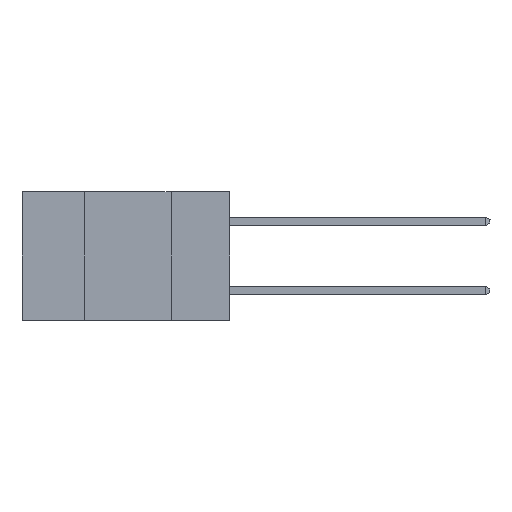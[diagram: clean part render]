
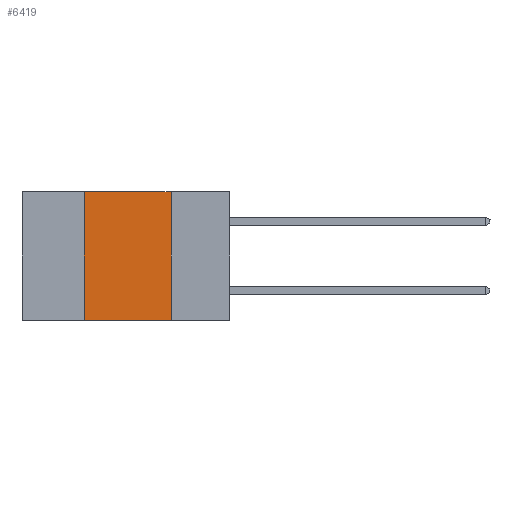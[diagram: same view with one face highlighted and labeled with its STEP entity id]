
A CAD part, left-side view. The second image highlights one B-rep face of the part: STEP entity #6419.
In plain terms, the highlighted planar face has unit normal (-1, 0, 0).
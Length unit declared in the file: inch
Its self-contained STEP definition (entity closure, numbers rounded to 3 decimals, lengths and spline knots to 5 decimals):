
#238 = EDGE_LOOP ( 'NONE', ( #22168, #12930, #23128, #16556 ) ) ;
#379 = LINE ( 'NONE', #8680, #2944 ) ;
#1309 = CARTESIAN_POINT ( 'NONE',  ( 0., 0.42, -0.37 ) ) ;
#1664 = CARTESIAN_POINT ( 'NONE',  ( 0., 0.17, -0.37 ) ) ;
#2242 = EDGE_CURVE ( 'NONE', #11374, #11615, #15884, .T. ) ;
#2944 = VECTOR ( 'NONE', #8531, 39.37008 ) ;
#3778 = DIRECTION ( 'NONE',  ( 0., -1., 0. ) ) ;
#4526 = EDGE_CURVE ( 'NONE', #20622, #18560, #5500, .T. ) ;
#4681 = DIRECTION ( 'NONE',  ( 0., 0., 1. ) ) ;
#5164 = DIRECTION ( 'NONE',  ( 0., 0., -1. ) ) ;
#5500 = LINE ( 'NONE', #20029, #12405 ) ;
#6259 = CARTESIAN_POINT ( 'NONE',  ( 0., 0.17, 0. ) ) ;
#6419 = ADVANCED_FACE ( 'NONE', ( #12013 ), #8944, .F. ) ;
#6427 = LINE ( 'NONE', #17594, #14457 ) ;
#8531 = DIRECTION ( 'NONE',  ( 0., 0., -1. ) ) ;
#8680 = CARTESIAN_POINT ( 'NONE',  ( 0., 0.17, 0. ) ) ;
#8944 = PLANE ( 'NONE',  #12514 ) ;
#9099 = DIRECTION ( 'NONE',  ( 1., 0., 0. ) ) ;
#9232 = DIRECTION ( 'NONE',  ( 0., -1., 0. ) ) ;
#11374 = VERTEX_POINT ( 'NONE', #21495 ) ;
#11615 = VERTEX_POINT ( 'NONE', #6259 ) ;
#12013 = FACE_OUTER_BOUND ( 'NONE', #238, .T. ) ;
#12405 = VECTOR ( 'NONE', #9232, 39.37008 ) ;
#12514 = AXIS2_PLACEMENT_3D ( 'NONE', #23565, #9099, #5164 ) ;
#12930 = ORIENTED_EDGE ( 'NONE', *, *, #2242, .F. ) ;
#14457 = VECTOR ( 'NONE', #4681, 39.37008 ) ;
#15884 = LINE ( 'NONE', #20102, #20142 ) ;
#16556 = ORIENTED_EDGE ( 'NONE', *, *, #4526, .T. ) ;
#17594 = CARTESIAN_POINT ( 'NONE',  ( 0., 0.42, 0. ) ) ;
#18560 = VERTEX_POINT ( 'NONE', #1664 ) ;
#18895 = EDGE_CURVE ( 'NONE', #11615, #18560, #379, .T. ) ;
#20029 = CARTESIAN_POINT ( 'NONE',  ( 0., 0.6, -0.37 ) ) ;
#20102 = CARTESIAN_POINT ( 'NONE',  ( 0., 0.6, 0. ) ) ;
#20142 = VECTOR ( 'NONE', #3778, 39.37008 ) ;
#20622 = VERTEX_POINT ( 'NONE', #1309 ) ;
#21495 = CARTESIAN_POINT ( 'NONE',  ( 0., 0.42, 0. ) ) ;
#22168 = ORIENTED_EDGE ( 'NONE', *, *, #18895, .F. ) ;
#22189 = EDGE_CURVE ( 'NONE', #20622, #11374, #6427, .T. ) ;
#23128 = ORIENTED_EDGE ( 'NONE', *, *, #22189, .F. ) ;
#23565 = CARTESIAN_POINT ( 'NONE',  ( 0., 0.6, 0. ) ) ;
